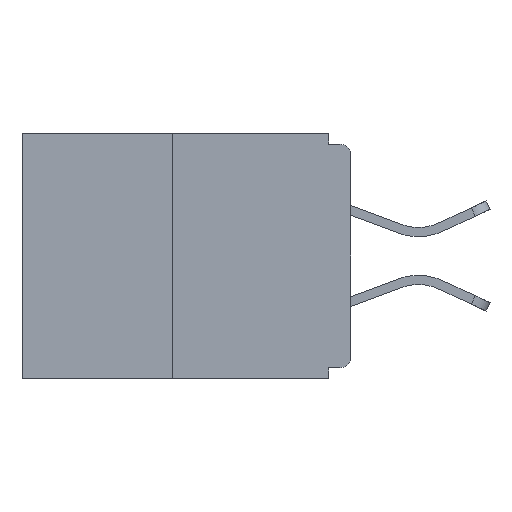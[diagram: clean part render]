
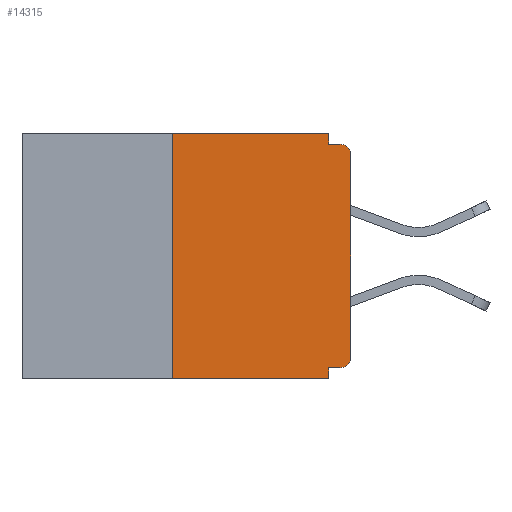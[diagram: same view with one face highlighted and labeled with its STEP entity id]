
A CAD part, left-side view. The second image highlights one B-rep face of the part: STEP entity #14315.
In plain terms, the highlighted planar face has unit normal (-1, 0, 0).
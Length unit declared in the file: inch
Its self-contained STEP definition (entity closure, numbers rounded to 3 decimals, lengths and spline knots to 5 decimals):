
#291 = DIRECTION ( 'NONE',  ( 0., 0., -1. ) ) ;
#370 = ORIENTED_EDGE ( 'NONE', *, *, #12717, .F. ) ;
#584 = CARTESIAN_POINT ( 'NONE',  ( 0., 0., -0.015 ) ) ;
#609 = LINE ( 'NONE', #5801, #25584 ) ;
#921 = CARTESIAN_POINT ( 'NONE',  ( 0., 0.015, -0.328 ) ) ;
#1059 = EDGE_CURVE ( 'NONE', #7923, #16664, #14610, .T. ) ;
#1469 = EDGE_CURVE ( 'NONE', #4574, #14734, #3537, .T. ) ;
#2252 = VECTOR ( 'NONE', #291, 39.37008 ) ;
#2561 = VECTOR ( 'NONE', #7693, 39.37008 ) ;
#3400 = AXIS2_PLACEMENT_3D ( 'NONE', #17982, #20045, #23886 ) ;
#3537 = LINE ( 'NONE', #26213, #2561 ) ;
#3803 = CARTESIAN_POINT ( 'NONE',  ( 0., 0., -0.328 ) ) ;
#3983 = VECTOR ( 'NONE', #14779, 39.37008 ) ;
#4354 = DIRECTION ( 'NONE',  ( 0., 0., -1. ) ) ;
#4406 = DIRECTION ( 'NONE',  ( -1., 0., 0. ) ) ;
#4426 = ORIENTED_EDGE ( 'NONE', *, *, #17223, .T. ) ;
#4574 = VERTEX_POINT ( 'NONE', #13372 ) ;
#5162 = CIRCLE ( 'NONE', #23179, 0.015 ) ;
#5801 = CARTESIAN_POINT ( 'NONE',  ( 0., 0.46, 0. ) ) ;
#5805 = DIRECTION ( 'NONE',  ( 0., 1., 0. ) ) ;
#5816 = VERTEX_POINT ( 'NONE', #19301 ) ;
#6151 = CARTESIAN_POINT ( 'NONE',  ( 0., 0.031, -0.015 ) ) ;
#6209 = VERTEX_POINT ( 'NONE', #20060 ) ;
#6516 = DIRECTION ( 'NONE',  ( -1., 0., 0. ) ) ;
#6562 = CARTESIAN_POINT ( 'NONE',  ( 0., 0.015, -0.313 ) ) ;
#7253 = LINE ( 'NONE', #23051, #22191 ) ;
#7605 = VERTEX_POINT ( 'NONE', #14051 ) ;
#7693 = DIRECTION ( 'NONE',  ( 0., -1., 0. ) ) ;
#7923 = VERTEX_POINT ( 'NONE', #24095 ) ;
#8578 = CARTESIAN_POINT ( 'NONE',  ( 0., 0.015, -0.03 ) ) ;
#9130 = ORIENTED_EDGE ( 'NONE', *, *, #1469, .T. ) ;
#9164 = ORIENTED_EDGE ( 'NONE', *, *, #11078, .F. ) ;
#9532 = ORIENTED_EDGE ( 'NONE', *, *, #22699, .F. ) ;
#9888 = VERTEX_POINT ( 'NONE', #13769 ) ;
#9995 = CARTESIAN_POINT ( 'NONE',  ( 0., 0.25, 0. ) ) ;
#10551 = LINE ( 'NONE', #9995, #11870 ) ;
#10685 = CARTESIAN_POINT ( 'NONE',  ( 0., 0.031, -0.343 ) ) ;
#11078 = EDGE_CURVE ( 'NONE', #4574, #6209, #10551, .T. ) ;
#11388 = LINE ( 'NONE', #3803, #18570 ) ;
#11870 = VECTOR ( 'NONE', #26344, 39.37008 ) ;
#11887 = EDGE_CURVE ( 'NONE', #7605, #14734, #7253, .T. ) ;
#12629 = DIRECTION ( 'NONE',  ( 0., 0., -1. ) ) ;
#12717 = EDGE_CURVE ( 'NONE', #16664, #21049, #13059, .T. ) ;
#13059 = LINE ( 'NONE', #584, #3983 ) ;
#13086 = ORIENTED_EDGE ( 'NONE', *, *, #15705, .T. ) ;
#13123 = ORIENTED_EDGE ( 'NONE', *, *, #11887, .F. ) ;
#13372 = CARTESIAN_POINT ( 'NONE',  ( 0., 0.25, -0.343 ) ) ;
#13689 = DIRECTION ( 'NONE',  ( 0., -1., 0. ) ) ;
#13769 = CARTESIAN_POINT ( 'NONE',  ( 0., 0., -0.313 ) ) ;
#13830 = EDGE_CURVE ( 'NONE', #19911, #9888, #5162, .T. ) ;
#13853 = CARTESIAN_POINT ( 'NONE',  ( 0., 0.015, -0.015 ) ) ;
#13923 = FACE_OUTER_BOUND ( 'NONE', #17126, .T. ) ;
#14051 = CARTESIAN_POINT ( 'NONE',  ( 0., 0.031, -0.328 ) ) ;
#14315 = ADVANCED_FACE ( 'NONE', ( #13923 ), #15634, .F. ) ;
#14610 = LINE ( 'NONE', #23058, #2252 ) ;
#14734 = VERTEX_POINT ( 'NONE', #10685 ) ;
#14779 = DIRECTION ( 'NONE',  ( 0., -1., 0. ) ) ;
#15419 = VECTOR ( 'NONE', #23420, 39.37008 ) ;
#15589 = ORIENTED_EDGE ( 'NONE', *, *, #1059, .F. ) ;
#15634 = PLANE ( 'NONE',  #3400 ) ;
#15705 = EDGE_CURVE ( 'NONE', #9888, #5816, #18912, .T. ) ;
#16612 = CARTESIAN_POINT ( 'NONE',  ( 0., 0., 0. ) ) ;
#16664 = VERTEX_POINT ( 'NONE', #6151 ) ;
#16688 = ORIENTED_EDGE ( 'NONE', *, *, #13830, .T. ) ;
#17126 = EDGE_LOOP ( 'NONE', ( #22786, #9164, #9130, #13123, #9532, #16688, #13086, #4426, #370, #15589 ) ) ;
#17223 = EDGE_CURVE ( 'NONE', #5816, #21049, #26022, .T. ) ;
#17982 = CARTESIAN_POINT ( 'NONE',  ( 0., 0.46, 0. ) ) ;
#18570 = VECTOR ( 'NONE', #5805, 39.37008 ) ;
#18912 = LINE ( 'NONE', #16612, #15419 ) ;
#19175 = EDGE_CURVE ( 'NONE', #6209, #7923, #609, .T. ) ;
#19301 = CARTESIAN_POINT ( 'NONE',  ( 0., 0., -0.03 ) ) ;
#19911 = VERTEX_POINT ( 'NONE', #921 ) ;
#20045 = DIRECTION ( 'NONE',  ( 1., 0., 0. ) ) ;
#20060 = CARTESIAN_POINT ( 'NONE',  ( 0., 0.25, 0. ) ) ;
#21049 = VERTEX_POINT ( 'NONE', #13853 ) ;
#22191 = VECTOR ( 'NONE', #12629, 39.37008 ) ;
#22699 = EDGE_CURVE ( 'NONE', #19911, #7605, #11388, .T. ) ;
#22786 = ORIENTED_EDGE ( 'NONE', *, *, #19175, .F. ) ;
#23051 = CARTESIAN_POINT ( 'NONE',  ( 0., 0.031, -0.343 ) ) ;
#23058 = CARTESIAN_POINT ( 'NONE',  ( 0., 0.031, 0. ) ) ;
#23157 = DIRECTION ( 'NONE',  ( 0., 0., -1. ) ) ;
#23179 = AXIS2_PLACEMENT_3D ( 'NONE', #6562, #4406, #23157 ) ;
#23420 = DIRECTION ( 'NONE',  ( 0., 0., 1. ) ) ;
#23886 = DIRECTION ( 'NONE',  ( 0., 0., -1. ) ) ;
#24095 = CARTESIAN_POINT ( 'NONE',  ( 0., 0.031, 0. ) ) ;
#25507 = AXIS2_PLACEMENT_3D ( 'NONE', #8578, #6516, #4354 ) ;
#25584 = VECTOR ( 'NONE', #13689, 39.37008 ) ;
#26022 = CIRCLE ( 'NONE', #25507, 0.015 ) ;
#26213 = CARTESIAN_POINT ( 'NONE',  ( 0., 0.46, -0.343 ) ) ;
#26344 = DIRECTION ( 'NONE',  ( 0., 0., 1. ) ) ;
